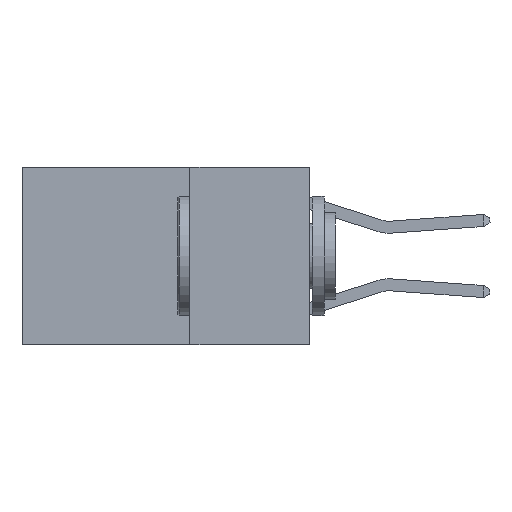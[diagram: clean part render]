
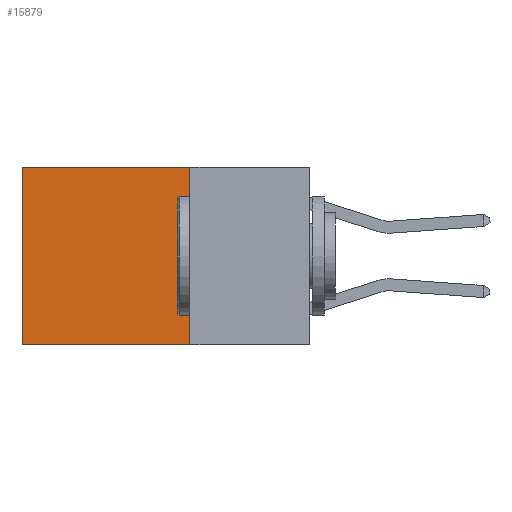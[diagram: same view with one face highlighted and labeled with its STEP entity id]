
A CAD part, left-side view. The second image highlights one B-rep face of the part: STEP entity #15879.
In plain terms, the highlighted planar face has unit normal (-1, 0, 0).
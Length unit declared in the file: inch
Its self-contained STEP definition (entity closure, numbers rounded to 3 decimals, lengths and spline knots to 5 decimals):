
#70 = CARTESIAN_POINT ( 'NONE',  ( 0.2625, 0.25, 0. ) ) ;
#754 = LINE ( 'NONE', #18992, #8906 ) ;
#810 = EDGE_LOOP ( 'NONE', ( #4697, #15085, #14552, #11879 ) ) ;
#1473 = CARTESIAN_POINT ( 'NONE',  ( 0.2625, 0.6, 0. ) ) ;
#2165 = CARTESIAN_POINT ( 'NONE',  ( 0.2625, 0.25, 0. ) ) ;
#4630 = AXIS2_PLACEMENT_3D ( 'NONE', #9006, #20217, #10620 ) ;
#4697 = ORIENTED_EDGE ( 'NONE', *, *, #5561, .T. ) ;
#5561 = EDGE_CURVE ( 'NONE', #6374, #20475, #9983, .T. ) ;
#5688 = VECTOR ( 'NONE', #8436, 39.37008 ) ;
#6374 = VERTEX_POINT ( 'NONE', #1473 ) ;
#6413 = CARTESIAN_POINT ( 'NONE',  ( 0.2625, 0.25, -0.37 ) ) ;
#7387 = VECTOR ( 'NONE', #17997, 39.37008 ) ;
#7890 = LINE ( 'NONE', #16396, #7387 ) ;
#8436 = DIRECTION ( 'NONE',  ( 0., 0., -1. ) ) ;
#8906 = VECTOR ( 'NONE', #20626, 39.37008 ) ;
#8967 = FACE_OUTER_BOUND ( 'NONE', #810, .T. ) ;
#9006 = CARTESIAN_POINT ( 'NONE',  ( 0.2625, 0.25, 0. ) ) ;
#9451 = VERTEX_POINT ( 'NONE', #6413 ) ;
#9983 = LINE ( 'NONE', #13204, #5688 ) ;
#10158 = VERTEX_POINT ( 'NONE', #70 ) ;
#10620 = DIRECTION ( 'NONE',  ( 0., 0., -1. ) ) ;
#10661 = EDGE_CURVE ( 'NONE', #10158, #6374, #754, .T. ) ;
#11028 = CARTESIAN_POINT ( 'NONE',  ( 0.2625, 0.6, -0.37 ) ) ;
#11045 = LINE ( 'NONE', #2165, #19043 ) ;
#11879 = ORIENTED_EDGE ( 'NONE', *, *, #10661, .T. ) ;
#13204 = CARTESIAN_POINT ( 'NONE',  ( 0.2625, 0.6, 0. ) ) ;
#14552 = ORIENTED_EDGE ( 'NONE', *, *, #20077, .F. ) ;
#15085 = ORIENTED_EDGE ( 'NONE', *, *, #16857, .F. ) ;
#15879 = ADVANCED_FACE ( 'NONE', ( #8967 ), #18601, .F. ) ;
#16396 = CARTESIAN_POINT ( 'NONE',  ( 0.2625, 0.25, -0.37 ) ) ;
#16628 = DIRECTION ( 'NONE',  ( 0., 0., -1. ) ) ;
#16857 = EDGE_CURVE ( 'NONE', #9451, #20475, #7890, .T. ) ;
#17997 = DIRECTION ( 'NONE',  ( 0., 1., 0. ) ) ;
#18601 = PLANE ( 'NONE',  #4630 ) ;
#18992 = CARTESIAN_POINT ( 'NONE',  ( 0.2625, 0.25, 0. ) ) ;
#19043 = VECTOR ( 'NONE', #16628, 39.37008 ) ;
#20077 = EDGE_CURVE ( 'NONE', #10158, #9451, #11045, .T. ) ;
#20217 = DIRECTION ( 'NONE',  ( 1., 0., 0. ) ) ;
#20475 = VERTEX_POINT ( 'NONE', #11028 ) ;
#20626 = DIRECTION ( 'NONE',  ( 0., 1., 0. ) ) ;
